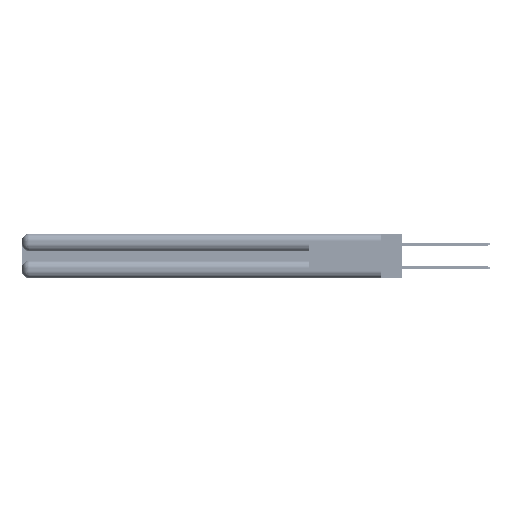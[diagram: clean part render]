
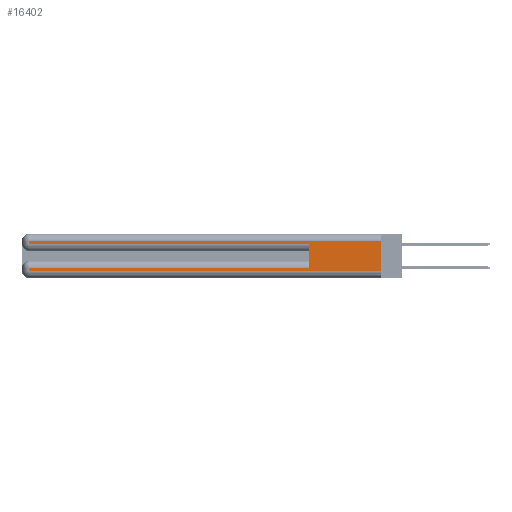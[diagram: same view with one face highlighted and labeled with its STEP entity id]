
A CAD part, left-side view. The second image highlights one B-rep face of the part: STEP entity #16402.
In plain terms, the highlighted planar face has unit normal (-1, 0, 0).
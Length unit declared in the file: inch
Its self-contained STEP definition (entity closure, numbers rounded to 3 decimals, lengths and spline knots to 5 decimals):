
#770 = VECTOR ( 'NONE', #12534, 39.37008 ) ;
#1312 = EDGE_CURVE ( 'NONE', #33441, #6380, #8598, .T. ) ;
#3305 = ORIENTED_EDGE ( 'NONE', *, *, #16398, .F. ) ;
#3751 = ORIENTED_EDGE ( 'NONE', *, *, #4677, .T. ) ;
#4078 = ORIENTED_EDGE ( 'NONE', *, *, #8611, .T. ) ;
#4677 = EDGE_CURVE ( 'NONE', #36934, #16923, #40036, .T. ) ;
#4699 = DIRECTION ( 'NONE',  ( 0., 0., 1. ) ) ;
#6380 = VERTEX_POINT ( 'NONE', #23210 ) ;
#7533 = DIRECTION ( 'NONE',  ( 0., -1., 0. ) ) ;
#7541 = CARTESIAN_POINT ( 'NONE',  ( 0., 0., 0.06 ) ) ;
#8598 = LINE ( 'NONE', #36575, #39586 ) ;
#8611 = EDGE_CURVE ( 'NONE', #16923, #28266, #9287, .T. ) ;
#8774 = CARTESIAN_POINT ( 'NONE',  ( 0., 2.94, 0.31 ) ) ;
#9014 = PLANE ( 'NONE',  #23738 ) ;
#9287 = LINE ( 'NONE', #24315, #49988 ) ;
#11821 = DIRECTION ( 'NONE',  ( 0., -1., 0. ) ) ;
#12534 = DIRECTION ( 'NONE',  ( 0., 1., 0. ) ) ;
#12785 = EDGE_LOOP ( 'NONE', ( #29995, #33375, #3751, #4078, #3305, #29948, #25337, #28462 ) ) ;
#14831 = CARTESIAN_POINT ( 'NONE',  ( 0., 0., 0.37 ) ) ;
#15838 = CARTESIAN_POINT ( 'NONE',  ( 0., 0.6, 0.285 ) ) ;
#16328 = EDGE_CURVE ( 'NONE', #46647, #33441, #45700, .T. ) ;
#16354 = CARTESIAN_POINT ( 'NONE',  ( 0., 2.94, 0.285 ) ) ;
#16398 = EDGE_CURVE ( 'NONE', #46647, #28266, #52825, .T. ) ;
#16402 = ADVANCED_FACE ( 'NONE', ( #44403 ), #9014, .F. ) ;
#16923 = VERTEX_POINT ( 'NONE', #16354 ) ;
#17497 = DIRECTION ( 'NONE',  ( 0., 0., -1. ) ) ;
#17689 = DIRECTION ( 'NONE',  ( 0., 0., -1. ) ) ;
#17750 = LINE ( 'NONE', #26553, #38837 ) ;
#18263 = DIRECTION ( 'NONE',  ( 0., 1., 0. ) ) ;
#20081 = CARTESIAN_POINT ( 'NONE',  ( 0., 0., 0.31 ) ) ;
#20851 = VECTOR ( 'NONE', #11821, 39.37008 ) ;
#21495 = CARTESIAN_POINT ( 'NONE',  ( 0., 2.94, 0.085 ) ) ;
#21916 = CARTESIAN_POINT ( 'NONE',  ( 0., 2.94, 0.37 ) ) ;
#22050 = LINE ( 'NONE', #14831, #52864 ) ;
#22271 = EDGE_CURVE ( 'NONE', #6380, #23125, #54275, .T. ) ;
#23125 = VERTEX_POINT ( 'NONE', #31302 ) ;
#23210 = CARTESIAN_POINT ( 'NONE',  ( 0., 2.94, 0.06 ) ) ;
#23738 = AXIS2_PLACEMENT_3D ( 'NONE', #38472, #42689, #17497 ) ;
#24315 = CARTESIAN_POINT ( 'NONE',  ( 0., 0., 0.285 ) ) ;
#25337 = ORIENTED_EDGE ( 'NONE', *, *, #1312, .T. ) ;
#26553 = CARTESIAN_POINT ( 'NONE',  ( 0., 0., 0.31 ) ) ;
#26704 = CARTESIAN_POINT ( 'NONE',  ( 0., 0.6, 0.085 ) ) ;
#27539 = VECTOR ( 'NONE', #17689, 39.37008 ) ;
#28266 = VERTEX_POINT ( 'NONE', #15838 ) ;
#28462 = ORIENTED_EDGE ( 'NONE', *, *, #22271, .T. ) ;
#29948 = ORIENTED_EDGE ( 'NONE', *, *, #16328, .T. ) ;
#29995 = ORIENTED_EDGE ( 'NONE', *, *, #44019, .F. ) ;
#30626 = VECTOR ( 'NONE', #4699, 39.37008 ) ;
#31302 = CARTESIAN_POINT ( 'NONE',  ( 0., 0., 0.06 ) ) ;
#31614 = DIRECTION ( 'NONE',  ( 0., 0., -1. ) ) ;
#33360 = CARTESIAN_POINT ( 'NONE',  ( 0., 0., 0.085 ) ) ;
#33375 = ORIENTED_EDGE ( 'NONE', *, *, #51643, .T. ) ;
#33441 = VERTEX_POINT ( 'NONE', #21495 ) ;
#36575 = CARTESIAN_POINT ( 'NONE',  ( 0., 2.94, 0.37 ) ) ;
#36934 = VERTEX_POINT ( 'NONE', #8774 ) ;
#38472 = CARTESIAN_POINT ( 'NONE',  ( 0., 0., 0.37 ) ) ;
#38837 = VECTOR ( 'NONE', #18263, 39.37008 ) ;
#39586 = VECTOR ( 'NONE', #49164, 39.37008 ) ;
#40036 = LINE ( 'NONE', #21916, #27539 ) ;
#42321 = CARTESIAN_POINT ( 'NONE',  ( 0., 0.6, 0.145 ) ) ;
#42689 = DIRECTION ( 'NONE',  ( 1., 0., 0. ) ) ;
#44019 = EDGE_CURVE ( 'NONE', #44857, #23125, #22050, .T. ) ;
#44403 = FACE_OUTER_BOUND ( 'NONE', #12785, .T. ) ;
#44857 = VERTEX_POINT ( 'NONE', #20081 ) ;
#45700 = LINE ( 'NONE', #33360, #770 ) ;
#46647 = VERTEX_POINT ( 'NONE', #26704 ) ;
#49164 = DIRECTION ( 'NONE',  ( 0., 0., -1. ) ) ;
#49988 = VECTOR ( 'NONE', #7533, 39.37008 ) ;
#51643 = EDGE_CURVE ( 'NONE', #44857, #36934, #17750, .T. ) ;
#52825 = LINE ( 'NONE', #42321, #30626 ) ;
#52864 = VECTOR ( 'NONE', #31614, 39.37008 ) ;
#54275 = LINE ( 'NONE', #7541, #20851 ) ;
